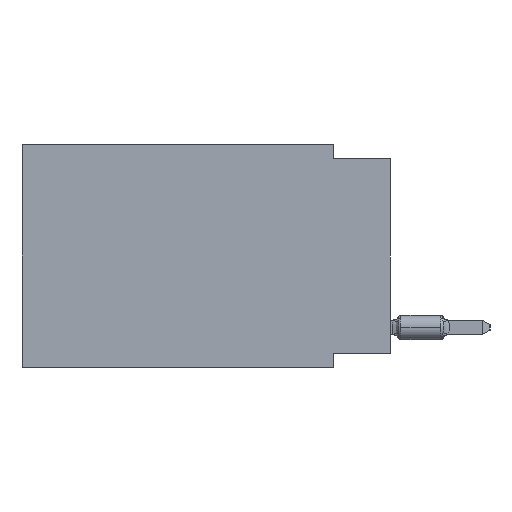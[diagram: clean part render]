
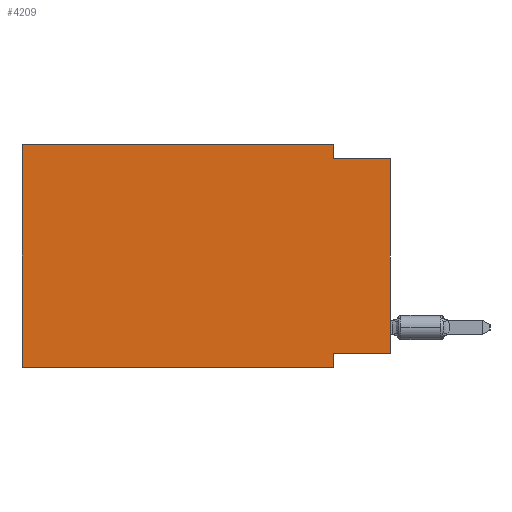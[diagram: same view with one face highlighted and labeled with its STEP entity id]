
A CAD part, left-side view. The second image highlights one B-rep face of the part: STEP entity #4209.
In plain terms, the highlighted planar face has unit normal (-1, 0, 0).
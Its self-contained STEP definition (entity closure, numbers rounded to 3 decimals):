
#179 = VECTOR ( 'NONE', #15688, 1000. ) ;
#821 = ORIENTED_EDGE ( 'NONE', *, *, #20847, .T. ) ;
#895 = DIRECTION ( 'NONE',  ( 0., 0., 1. ) ) ;
#1714 = ORIENTED_EDGE ( 'NONE', *, *, #10884, .F. ) ;
#2330 = ORIENTED_EDGE ( 'NONE', *, *, #36888, .T. ) ;
#3414 = CARTESIAN_POINT ( 'NONE',  ( 0., 2.54, -0.635 ) ) ;
#3876 = EDGE_CURVE ( 'NONE', #23873, #23276, #32854, .T. ) ;
#4209 = ADVANCED_FACE ( 'NONE', ( #15452 ), #38700, .F. ) ;
#4308 = DIRECTION ( 'NONE',  ( 0., 0., 1. ) ) ;
#4650 = VECTOR ( 'NONE', #13930, 1000. ) ;
#5149 = DIRECTION ( 'NONE',  ( 0., 0., -1. ) ) ;
#5662 = CARTESIAN_POINT ( 'NONE',  ( 0., 2.54, -9.906 ) ) ;
#5980 = VERTEX_POINT ( 'NONE', #36661 ) ;
#7433 = VERTEX_POINT ( 'NONE', #48038 ) ;
#10884 = EDGE_CURVE ( 'NONE', #31786, #23873, #43866, .T. ) ;
#11807 = ORIENTED_EDGE ( 'NONE', *, *, #27431, .F. ) ;
#13930 = DIRECTION ( 'NONE',  ( 0., 1., 0. ) ) ;
#15452 = FACE_OUTER_BOUND ( 'NONE', #18046, .T. ) ;
#15688 = DIRECTION ( 'NONE',  ( 0., -1., 0. ) ) ;
#15752 = ORIENTED_EDGE ( 'NONE', *, *, #3876, .F. ) ;
#16073 = VECTOR ( 'NONE', #20404, 1000. ) ;
#17412 = LINE ( 'NONE', #5662, #44390 ) ;
#18046 = EDGE_LOOP ( 'NONE', ( #2330, #15752, #1714, #21995, #37975, #821, #34630, #11807 ) ) ;
#18633 = LINE ( 'NONE', #26459, #179 ) ;
#18773 = LINE ( 'NONE', #33698, #32701 ) ;
#19696 = VERTEX_POINT ( 'NONE', #33803 ) ;
#20204 = DIRECTION ( 'NONE',  ( 0., -1., 0. ) ) ;
#20404 = DIRECTION ( 'NONE',  ( 0., 0., -1. ) ) ;
#20610 = DIRECTION ( 'NONE',  ( 0., 0., -1. ) ) ;
#20847 = EDGE_CURVE ( 'NONE', #5980, #36251, #18633, .T. ) ;
#21995 = ORIENTED_EDGE ( 'NONE', *, *, #27609, .F. ) ;
#23276 = VERTEX_POINT ( 'NONE', #34369 ) ;
#23526 = VECTOR ( 'NONE', #38388, 1000. ) ;
#23640 = CARTESIAN_POINT ( 'NONE',  ( 0., 0., -0.635 ) ) ;
#23873 = VERTEX_POINT ( 'NONE', #3414 ) ;
#23916 = LINE ( 'NONE', #31744, #23526 ) ;
#23992 = DIRECTION ( 'NONE',  ( 1., 0., 0. ) ) ;
#24661 = VECTOR ( 'NONE', #895, 1000. ) ;
#24777 = CARTESIAN_POINT ( 'NONE',  ( 0., 2.54, -9.906 ) ) ;
#26459 = CARTESIAN_POINT ( 'NONE',  ( 0., 16.383, -9.906 ) ) ;
#27431 = EDGE_CURVE ( 'NONE', #19696, #7433, #40604, .T. ) ;
#27457 = AXIS2_PLACEMENT_3D ( 'NONE', #31353, #23992, #5149 ) ;
#27577 = CARTESIAN_POINT ( 'NONE',  ( 0., 2.54, 0. ) ) ;
#27609 = EDGE_CURVE ( 'NONE', #41416, #31786, #23916, .T. ) ;
#31296 = VECTOR ( 'NONE', #20204, 1000. ) ;
#31353 = CARTESIAN_POINT ( 'NONE',  ( 0., 16.383, 0. ) ) ;
#31744 = CARTESIAN_POINT ( 'NONE',  ( 0., 16.383, 0. ) ) ;
#31786 = VERTEX_POINT ( 'NONE', #27577 ) ;
#32701 = VECTOR ( 'NONE', #4308, 1000. ) ;
#32854 = LINE ( 'NONE', #23640, #31296 ) ;
#33698 = CARTESIAN_POINT ( 'NONE',  ( 0., 0., 0. ) ) ;
#33803 = CARTESIAN_POINT ( 'NONE',  ( 0., 0., -9.271 ) ) ;
#34369 = CARTESIAN_POINT ( 'NONE',  ( 0., 0., -0.635 ) ) ;
#34630 = ORIENTED_EDGE ( 'NONE', *, *, #47141, .F. ) ;
#36251 = VERTEX_POINT ( 'NONE', #24777 ) ;
#36661 = CARTESIAN_POINT ( 'NONE',  ( 0., 16.383, -9.906 ) ) ;
#36888 = EDGE_CURVE ( 'NONE', #19696, #23276, #18773, .T. ) ;
#36933 = CARTESIAN_POINT ( 'NONE',  ( 0., 0., -9.271 ) ) ;
#37063 = CARTESIAN_POINT ( 'NONE',  ( 0., 16.383, 0. ) ) ;
#37975 = ORIENTED_EDGE ( 'NONE', *, *, #43945, .F. ) ;
#38361 = CARTESIAN_POINT ( 'NONE',  ( 0., 16.383, 0. ) ) ;
#38388 = DIRECTION ( 'NONE',  ( 0., -1., 0. ) ) ;
#38700 = PLANE ( 'NONE',  #27457 ) ;
#40203 = CARTESIAN_POINT ( 'NONE',  ( 0., 2.54, 0. ) ) ;
#40604 = LINE ( 'NONE', #36933, #4650 ) ;
#41416 = VERTEX_POINT ( 'NONE', #37063 ) ;
#42260 = LINE ( 'NONE', #38361, #24661 ) ;
#43866 = LINE ( 'NONE', #40203, #16073 ) ;
#43945 = EDGE_CURVE ( 'NONE', #5980, #41416, #42260, .T. ) ;
#44390 = VECTOR ( 'NONE', #20610, 1000. ) ;
#47141 = EDGE_CURVE ( 'NONE', #7433, #36251, #17412, .T. ) ;
#48038 = CARTESIAN_POINT ( 'NONE',  ( 0., 2.54, -9.271 ) ) ;
